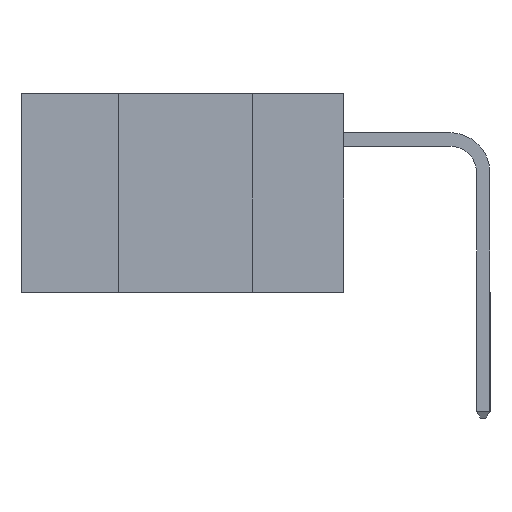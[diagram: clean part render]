
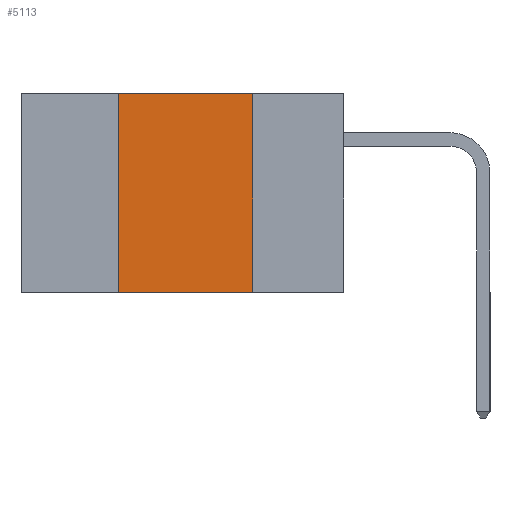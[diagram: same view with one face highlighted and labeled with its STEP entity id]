
A CAD part, left-side view. The second image highlights one B-rep face of the part: STEP entity #5113.
In plain terms, the highlighted planar face has unit normal (-1, 0, 0).
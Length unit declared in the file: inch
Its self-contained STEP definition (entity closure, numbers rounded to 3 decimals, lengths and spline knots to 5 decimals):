
#390 = DIRECTION ( 'NONE',  ( 0., -1., 0. ) ) ;
#1819 = DIRECTION ( 'NONE',  ( 0., -1., 0. ) ) ;
#2097 = ORIENTED_EDGE ( 'NONE', *, *, #7520, .F. ) ;
#2265 = LINE ( 'NONE', #5691, #9381 ) ;
#3105 = PLANE ( 'NONE',  #3766 ) ;
#3175 = VECTOR ( 'NONE', #9852, 39.37008 ) ;
#3392 = FACE_OUTER_BOUND ( 'NONE', #12207, .T. ) ;
#3635 = VECTOR ( 'NONE', #8216, 39.37008 ) ;
#3751 = ORIENTED_EDGE ( 'NONE', *, *, #7701, .F. ) ;
#3766 = AXIS2_PLACEMENT_3D ( 'NONE', #4071, #5064, #11684 ) ;
#3911 = ORIENTED_EDGE ( 'NONE', *, *, #6327, .T. ) ;
#4071 = CARTESIAN_POINT ( 'NONE',  ( 0., 0.6, 0. ) ) ;
#4182 = EDGE_CURVE ( 'NONE', #6951, #4329, #2265, .T. ) ;
#4215 = CARTESIAN_POINT ( 'NONE',  ( 0., 0.6, -0.37 ) ) ;
#4329 = VERTEX_POINT ( 'NONE', #4888 ) ;
#4888 = CARTESIAN_POINT ( 'NONE',  ( 0., 0.17, 0. ) ) ;
#5064 = DIRECTION ( 'NONE',  ( 1., 0., 0. ) ) ;
#5113 = ADVANCED_FACE ( 'NONE', ( #3392 ), #3105, .F. ) ;
#5691 = CARTESIAN_POINT ( 'NONE',  ( 0., 0.6, 0. ) ) ;
#6093 = CARTESIAN_POINT ( 'NONE',  ( 0., 0.42, 0. ) ) ;
#6327 = EDGE_CURVE ( 'NONE', #8162, #10524, #11850, .T. ) ;
#6535 = LINE ( 'NONE', #10996, #3635 ) ;
#6951 = VERTEX_POINT ( 'NONE', #6093 ) ;
#7520 = EDGE_CURVE ( 'NONE', #8162, #6951, #10832, .T. ) ;
#7701 = EDGE_CURVE ( 'NONE', #4329, #10524, #6535, .T. ) ;
#8162 = VERTEX_POINT ( 'NONE', #10034 ) ;
#8216 = DIRECTION ( 'NONE',  ( 0., 0., -1. ) ) ;
#8893 = CARTESIAN_POINT ( 'NONE',  ( 0., 0.42, 0. ) ) ;
#9381 = VECTOR ( 'NONE', #1819, 39.37008 ) ;
#9412 = VECTOR ( 'NONE', #390, 39.37008 ) ;
#9852 = DIRECTION ( 'NONE',  ( 0., 0., 1. ) ) ;
#10034 = CARTESIAN_POINT ( 'NONE',  ( 0., 0.42, -0.37 ) ) ;
#10524 = VERTEX_POINT ( 'NONE', #11962 ) ;
#10832 = LINE ( 'NONE', #8893, #3175 ) ;
#10996 = CARTESIAN_POINT ( 'NONE',  ( 0., 0.17, 0. ) ) ;
#11684 = DIRECTION ( 'NONE',  ( 0., 0., -1. ) ) ;
#11850 = LINE ( 'NONE', #4215, #9412 ) ;
#11935 = ORIENTED_EDGE ( 'NONE', *, *, #4182, .F. ) ;
#11962 = CARTESIAN_POINT ( 'NONE',  ( 0., 0.17, -0.37 ) ) ;
#12207 = EDGE_LOOP ( 'NONE', ( #3751, #11935, #2097, #3911 ) ) ;
